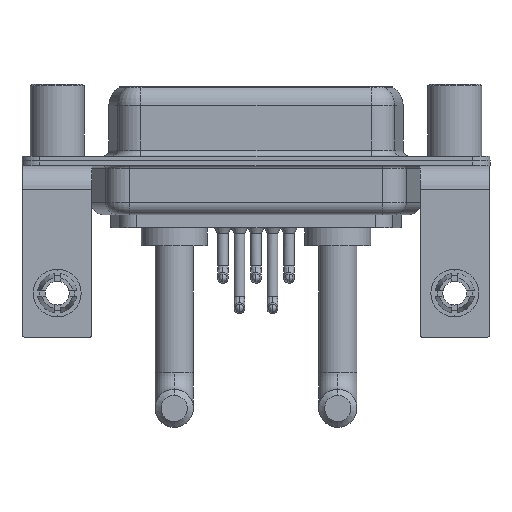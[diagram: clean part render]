
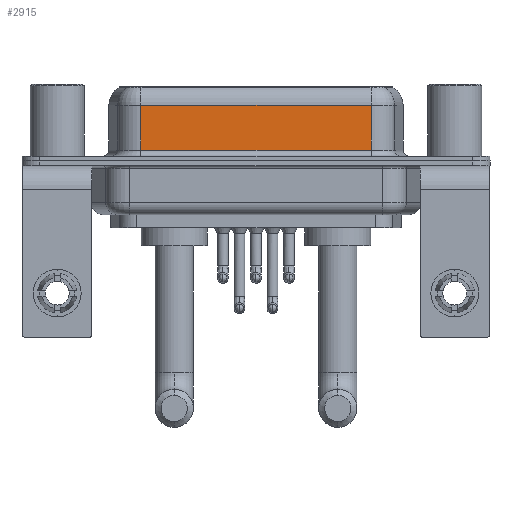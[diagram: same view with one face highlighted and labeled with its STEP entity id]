
A CAD part, front view. The second image highlights one B-rep face of the part: STEP entity #2915.
In plain terms, the highlighted planar face has unit normal (0, -1, 0).
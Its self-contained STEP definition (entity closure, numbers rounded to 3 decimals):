
#370 = CARTESIAN_POINT ( 'NONE',  ( 26.287, -3.95, 4.65 ) ) ;
#388 = CARTESIAN_POINT ( 'NONE',  ( 26.287, -3.95, 0.9 ) ) ;
#2009 = ORIENTED_EDGE ( 'NONE', *, *, #20180, .F. ) ;
#2283 = PLANE ( 'NONE',  #2880 ) ;
#2738 = CARTESIAN_POINT ( 'NONE',  ( 26.287, -3.95, 0.9 ) ) ;
#2880 = AXIS2_PLACEMENT_3D ( 'NONE', #4137, #10337, #8479 ) ;
#2915 = ADVANCED_FACE ( 'NONE', ( #14899 ), #2283, .F. ) ;
#4065 = VERTEX_POINT ( 'NONE', #9319 ) ;
#4137 = CARTESIAN_POINT ( 'NONE',  ( 26.287, -3.95, 6.4 ) ) ;
#5345 = VECTOR ( 'NONE', #14653, 1000. ) ;
#6474 = EDGE_CURVE ( 'NONE', #9282, #4065, #9589, .T. ) ;
#8479 = DIRECTION ( 'NONE',  ( 0., 0., 1. ) ) ;
#8556 = LINE ( 'NONE', #14872, #10412 ) ;
#8834 = LINE ( 'NONE', #388, #18223 ) ;
#9282 = VERTEX_POINT ( 'NONE', #14031 ) ;
#9319 = CARTESIAN_POINT ( 'NONE',  ( 7.013, -3.95, 4.65 ) ) ;
#9589 = LINE ( 'NONE', #370, #5345 ) ;
#10070 = VERTEX_POINT ( 'NONE', #13774 ) ;
#10337 = DIRECTION ( 'NONE',  ( 0., 1., 0. ) ) ;
#10412 = VECTOR ( 'NONE', #13418, 1000. ) ;
#10866 = VECTOR ( 'NONE', #13763, 1000. ) ;
#13418 = DIRECTION ( 'NONE',  ( 0., 0., -1. ) ) ;
#13660 = EDGE_CURVE ( 'NONE', #10070, #17881, #8834, .T. ) ;
#13763 = DIRECTION ( 'NONE',  ( 0., 0., -1. ) ) ;
#13774 = CARTESIAN_POINT ( 'NONE',  ( 7.013, -3.95, 0.9 ) ) ;
#14031 = CARTESIAN_POINT ( 'NONE',  ( 26.287, -3.95, 4.65 ) ) ;
#14653 = DIRECTION ( 'NONE',  ( -1., 0., 0. ) ) ;
#14872 = CARTESIAN_POINT ( 'NONE',  ( 7.013, -3.95, 6.4 ) ) ;
#14899 = FACE_OUTER_BOUND ( 'NONE', #17196, .T. ) ;
#14906 = LINE ( 'NONE', #15301, #10866 ) ;
#15109 = ORIENTED_EDGE ( 'NONE', *, *, #6474, .T. ) ;
#15147 = DIRECTION ( 'NONE',  ( 1., 0., 0. ) ) ;
#15301 = CARTESIAN_POINT ( 'NONE',  ( 26.287, -3.95, 6.4 ) ) ;
#16412 = ORIENTED_EDGE ( 'NONE', *, *, #16436, .T. ) ;
#16436 = EDGE_CURVE ( 'NONE', #4065, #10070, #8556, .T. ) ;
#17196 = EDGE_LOOP ( 'NONE', ( #2009, #15109, #16412, #17545 ) ) ;
#17545 = ORIENTED_EDGE ( 'NONE', *, *, #13660, .T. ) ;
#17881 = VERTEX_POINT ( 'NONE', #2738 ) ;
#18223 = VECTOR ( 'NONE', #15147, 1000. ) ;
#20180 = EDGE_CURVE ( 'NONE', #9282, #17881, #14906, .T. ) ;
